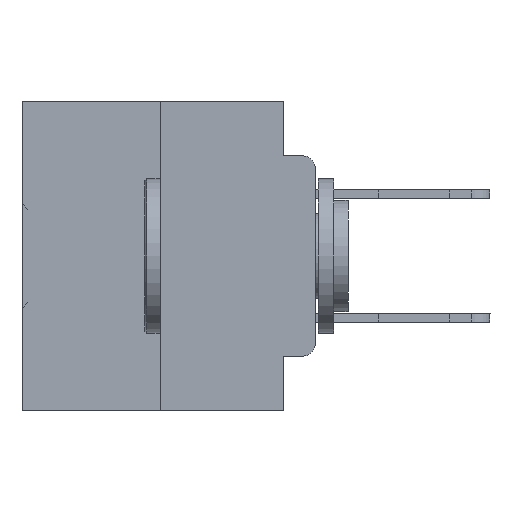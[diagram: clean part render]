
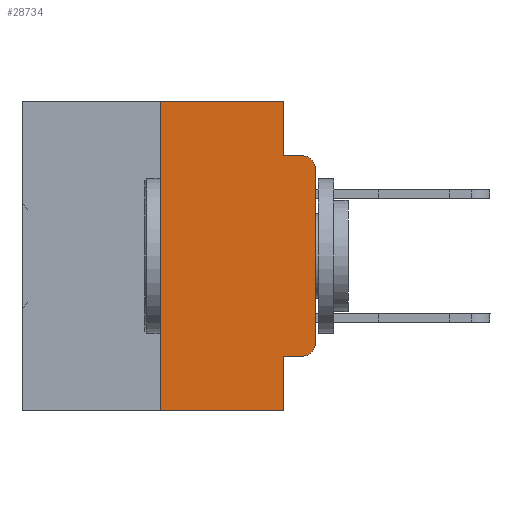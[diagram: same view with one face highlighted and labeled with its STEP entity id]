
A CAD part, left-side view. The second image highlights one B-rep face of the part: STEP entity #28734.
In plain terms, the highlighted planar face has unit normal (-1, 0, 0).
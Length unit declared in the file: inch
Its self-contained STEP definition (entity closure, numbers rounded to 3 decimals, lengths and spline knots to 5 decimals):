
#109 = CARTESIAN_POINT ( 'NONE',  ( 0., 0.473, 0. ) ) ;
#244 = ORIENTED_EDGE ( 'NONE', *, *, #2747, .T. ) ;
#743 = CARTESIAN_POINT ( 'NONE',  ( 0., 0.051, -0.0885 ) ) ;
#1560 = VERTEX_POINT ( 'NONE', #6631 ) ;
#2145 = CARTESIAN_POINT ( 'NONE',  ( 0., 0.473, -0.5 ) ) ;
#2298 = DIRECTION ( 'NONE',  ( 0., 0., 1. ) ) ;
#2747 = EDGE_CURVE ( 'NONE', #22982, #8856, #21353, .T. ) ;
#3101 = DIRECTION ( 'NONE',  ( 1., 0., 0. ) ) ;
#4225 = EDGE_CURVE ( 'NONE', #18593, #10356, #15820, .T. ) ;
#4735 = EDGE_CURVE ( 'NONE', #8856, #7533, #13991, .T. ) ;
#4908 = VECTOR ( 'NONE', #36363, 39.37008 ) ;
#5405 = ORIENTED_EDGE ( 'NONE', *, *, #32712, .F. ) ;
#6631 = CARTESIAN_POINT ( 'NONE',  ( 0., 0.051, -0.0885 ) ) ;
#6857 = DIRECTION ( 'NONE',  ( 0., 0., -1. ) ) ;
#7533 = VERTEX_POINT ( 'NONE', #12880 ) ;
#8024 = VECTOR ( 'NONE', #8100, 39.37008 ) ;
#8100 = DIRECTION ( 'NONE',  ( 0., -1., 0. ) ) ;
#8856 = VERTEX_POINT ( 'NONE', #15163 ) ;
#9845 = DIRECTION ( 'NONE',  ( -1., 0., 0. ) ) ;
#9850 = LINE ( 'NONE', #36923, #17602 ) ;
#10356 = VERTEX_POINT ( 'NONE', #24502 ) ;
#11284 = VERTEX_POINT ( 'NONE', #17531 ) ;
#11824 = FACE_OUTER_BOUND ( 'NONE', #35628, .T. ) ;
#12880 = CARTESIAN_POINT ( 'NONE',  ( 0., 0., -0.3915 ) ) ;
#13991 = CIRCLE ( 'NONE', #35772, 0.02 ) ;
#15163 = CARTESIAN_POINT ( 'NONE',  ( 0., 0.02, -0.4115 ) ) ;
#15516 = ORIENTED_EDGE ( 'NONE', *, *, #26917, .T. ) ;
#15600 = CARTESIAN_POINT ( 'NONE',  ( 0., 0.051, 0. ) ) ;
#15820 = LINE ( 'NONE', #2145, #8024 ) ;
#16120 = DIRECTION ( 'NONE',  ( -1., 0., 0. ) ) ;
#16261 = EDGE_CURVE ( 'NONE', #11284, #25357, #31307, .T. ) ;
#16491 = CARTESIAN_POINT ( 'NONE',  ( 0., 0.473, 0. ) ) ;
#16823 = DIRECTION ( 'NONE',  ( 0., 0., -1. ) ) ;
#16883 = VECTOR ( 'NONE', #19389, 39.37008 ) ;
#17066 = CARTESIAN_POINT ( 'NONE',  ( 0., 0.25, 0. ) ) ;
#17531 = CARTESIAN_POINT ( 'NONE',  ( 0., 0.25, 0. ) ) ;
#17602 = VECTOR ( 'NONE', #16823, 39.37008 ) ;
#17747 = PLANE ( 'NONE',  #31328 ) ;
#18179 = ORIENTED_EDGE ( 'NONE', *, *, #16261, .F. ) ;
#18593 = VERTEX_POINT ( 'NONE', #33944 ) ;
#19389 = DIRECTION ( 'NONE',  ( 0., -1., 0. ) ) ;
#19700 = LINE ( 'NONE', #17066, #35011 ) ;
#20900 = ORIENTED_EDGE ( 'NONE', *, *, #4225, .T. ) ;
#21120 = EDGE_CURVE ( 'NONE', #7533, #21733, #35756, .T. ) ;
#21254 = DIRECTION ( 'NONE',  ( 0., -1., 0. ) ) ;
#21353 = LINE ( 'NONE', #33533, #4908 ) ;
#21733 = VERTEX_POINT ( 'NONE', #24909 ) ;
#21808 = CARTESIAN_POINT ( 'NONE',  ( 0., 0.051, -0.4115 ) ) ;
#22636 = LINE ( 'NONE', #743, #29427 ) ;
#22982 = VERTEX_POINT ( 'NONE', #21808 ) ;
#23540 = DIRECTION ( 'NONE',  ( 0., 0., -1. ) ) ;
#23603 = VECTOR ( 'NONE', #6857, 39.37008 ) ;
#24498 = ORIENTED_EDGE ( 'NONE', *, *, #4735, .T. ) ;
#24502 = CARTESIAN_POINT ( 'NONE',  ( 0., 0.051, -0.5 ) ) ;
#24906 = CARTESIAN_POINT ( 'NONE',  ( 0., 0.02, -0.0885 ) ) ;
#24909 = CARTESIAN_POINT ( 'NONE',  ( 0., 0., -0.1085 ) ) ;
#25357 = VERTEX_POINT ( 'NONE', #26347 ) ;
#26347 = CARTESIAN_POINT ( 'NONE',  ( 0., 0.051, 0. ) ) ;
#26917 = EDGE_CURVE ( 'NONE', #21733, #36662, #28222, .T. ) ;
#27184 = CARTESIAN_POINT ( 'NONE',  ( 0., 0.02, -0.1085 ) ) ;
#27229 = ORIENTED_EDGE ( 'NONE', *, *, #21120, .T. ) ;
#27231 = VECTOR ( 'NONE', #36498, 39.37008 ) ;
#27664 = ORIENTED_EDGE ( 'NONE', *, *, #34636, .F. ) ;
#27708 = ORIENTED_EDGE ( 'NONE', *, *, #28874, .F. ) ;
#27873 = CARTESIAN_POINT ( 'NONE',  ( 0., 0., 0. ) ) ;
#28222 = CIRCLE ( 'NONE', #37012, 0.02 ) ;
#28734 = ADVANCED_FACE ( 'NONE', ( #11824 ), #17747, .F. ) ;
#28874 = EDGE_CURVE ( 'NONE', #1560, #36662, #22636, .T. ) ;
#29427 = VECTOR ( 'NONE', #21254, 39.37008 ) ;
#30104 = DIRECTION ( 'NONE',  ( 0., 0., -1. ) ) ;
#31267 = LINE ( 'NONE', #15600, #23603 ) ;
#31307 = LINE ( 'NONE', #16491, #16883 ) ;
#31328 = AXIS2_PLACEMENT_3D ( 'NONE', #109, #3101, #23540 ) ;
#32712 = EDGE_CURVE ( 'NONE', #25357, #1560, #9850, .T. ) ;
#33393 = CARTESIAN_POINT ( 'NONE',  ( 0., 0.02, -0.3915 ) ) ;
#33533 = CARTESIAN_POINT ( 'NONE',  ( 0., 0.051, -0.4115 ) ) ;
#33944 = CARTESIAN_POINT ( 'NONE',  ( 0., 0.25, -0.5 ) ) ;
#34636 = EDGE_CURVE ( 'NONE', #18593, #11284, #19700, .T. ) ;
#35011 = VECTOR ( 'NONE', #2298, 39.37008 ) ;
#35628 = EDGE_LOOP ( 'NONE', ( #27229, #15516, #27708, #5405, #18179, #27664, #20900, #36166, #244, #24498 ) ) ;
#35756 = LINE ( 'NONE', #27873, #27231 ) ;
#35772 = AXIS2_PLACEMENT_3D ( 'NONE', #33393, #16120, #36233 ) ;
#36166 = ORIENTED_EDGE ( 'NONE', *, *, #36520, .F. ) ;
#36233 = DIRECTION ( 'NONE',  ( 0., 0., -1. ) ) ;
#36363 = DIRECTION ( 'NONE',  ( 0., -1., 0. ) ) ;
#36498 = DIRECTION ( 'NONE',  ( 0., 0., 1. ) ) ;
#36520 = EDGE_CURVE ( 'NONE', #22982, #10356, #31267, .T. ) ;
#36662 = VERTEX_POINT ( 'NONE', #24906 ) ;
#36923 = CARTESIAN_POINT ( 'NONE',  ( 0., 0.051, 0. ) ) ;
#37012 = AXIS2_PLACEMENT_3D ( 'NONE', #27184, #9845, #30104 ) ;
